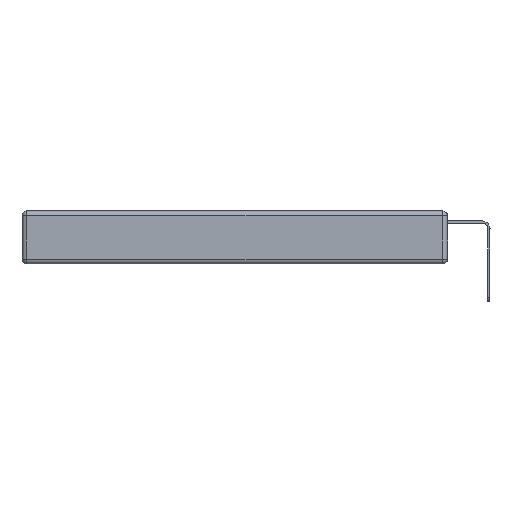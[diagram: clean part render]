
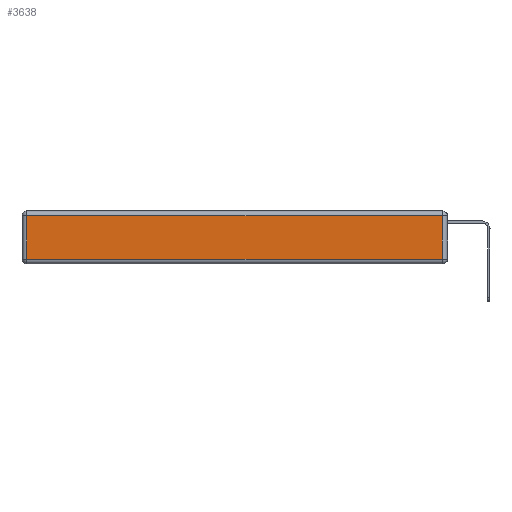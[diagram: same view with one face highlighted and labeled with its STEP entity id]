
A CAD part, left-side view. The second image highlights one B-rep face of the part: STEP entity #3638.
In plain terms, the highlighted planar face has unit normal (-1, 0, 0).
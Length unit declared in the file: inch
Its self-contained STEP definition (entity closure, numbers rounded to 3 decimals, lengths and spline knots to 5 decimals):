
#515 = EDGE_CURVE ( 'NONE', #10936, #3609, #11866, .T. ) ;
#1032 = VECTOR ( 'NONE', #3551, 39.37008 ) ;
#1090 = FACE_OUTER_BOUND ( 'NONE', #5795, .T. ) ;
#1186 = VECTOR ( 'NONE', #9911, 39.37008 ) ;
#1320 = VECTOR ( 'NONE', #6500, 39.37008 ) ;
#1355 = AXIS2_PLACEMENT_3D ( 'NONE', #7492, #6798, #9704 ) ;
#1504 = LINE ( 'NONE', #4371, #1032 ) ;
#1619 = VERTEX_POINT ( 'NONE', #12324 ) ;
#1802 = PLANE ( 'NONE',  #1355 ) ;
#2547 = CARTESIAN_POINT ( 'NONE',  ( 0., 2.75, -0.03 ) ) ;
#3077 = DIRECTION ( 'NONE',  ( 0., 0., -1. ) ) ;
#3551 = DIRECTION ( 'NONE',  ( 0., -1., 0. ) ) ;
#3609 = VERTEX_POINT ( 'NONE', #4728 ) ;
#3638 = ADVANCED_FACE ( 'NONE', ( #1090 ), #1802, .T. ) ;
#3876 = LINE ( 'NONE', #2547, #1320 ) ;
#4371 = CARTESIAN_POINT ( 'NONE',  ( 0., 0., -0.313 ) ) ;
#4728 = CARTESIAN_POINT ( 'NONE',  ( 0., 2.72, -0.313 ) ) ;
#5763 = ORIENTED_EDGE ( 'NONE', *, *, #11699, .T. ) ;
#5795 = EDGE_LOOP ( 'NONE', ( #5763, #10350, #8624, #10511 ) ) ;
#6500 = DIRECTION ( 'NONE',  ( 0., 1., 0. ) ) ;
#6798 = DIRECTION ( 'NONE',  ( -1., 0., 0. ) ) ;
#6835 = CARTESIAN_POINT ( 'NONE',  ( 0., 2.72, -0.343 ) ) ;
#6850 = VERTEX_POINT ( 'NONE', #10656 ) ;
#6892 = EDGE_CURVE ( 'NONE', #6850, #1619, #10660, .T. ) ;
#7483 = EDGE_CURVE ( 'NONE', #1619, #10936, #3876, .T. ) ;
#7492 = CARTESIAN_POINT ( 'NONE',  ( 0., 0., -0.343 ) ) ;
#8624 = ORIENTED_EDGE ( 'NONE', *, *, #7483, .T. ) ;
#8999 = CARTESIAN_POINT ( 'NONE',  ( 0., 2.72, -0.03 ) ) ;
#9704 = DIRECTION ( 'NONE',  ( 0., 0., 1. ) ) ;
#9911 = DIRECTION ( 'NONE',  ( 0., 0., 1. ) ) ;
#10350 = ORIENTED_EDGE ( 'NONE', *, *, #6892, .T. ) ;
#10511 = ORIENTED_EDGE ( 'NONE', *, *, #515, .T. ) ;
#10656 = CARTESIAN_POINT ( 'NONE',  ( 0., 0.03, -0.313 ) ) ;
#10660 = LINE ( 'NONE', #10746, #1186 ) ;
#10746 = CARTESIAN_POINT ( 'NONE',  ( 0., 0.03, -0.343 ) ) ;
#10936 = VERTEX_POINT ( 'NONE', #8999 ) ;
#11129 = VECTOR ( 'NONE', #3077, 39.37008 ) ;
#11699 = EDGE_CURVE ( 'NONE', #3609, #6850, #1504, .T. ) ;
#11866 = LINE ( 'NONE', #6835, #11129 ) ;
#12324 = CARTESIAN_POINT ( 'NONE',  ( 0., 0.03, -0.03 ) ) ;
